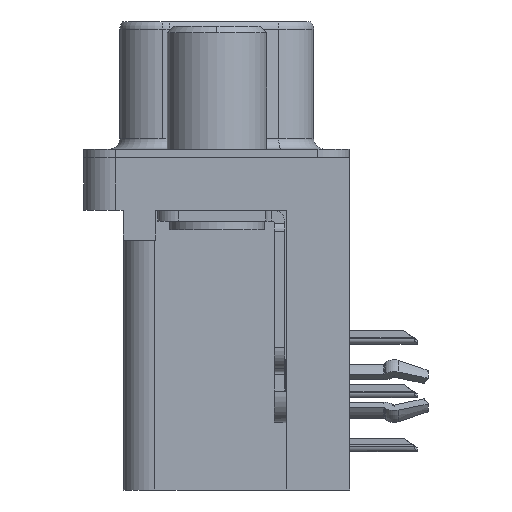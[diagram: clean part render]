
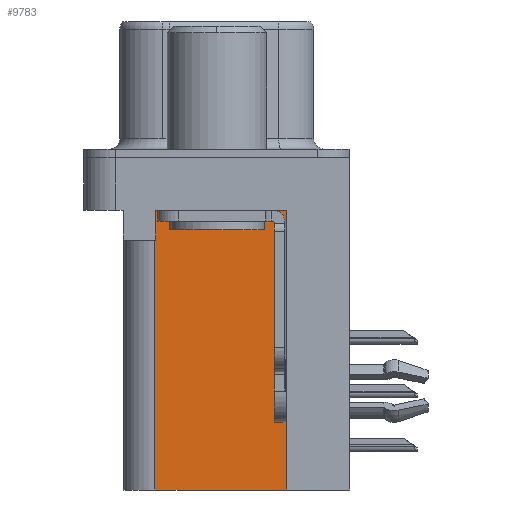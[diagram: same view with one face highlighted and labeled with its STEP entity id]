
A CAD part, left-side view. The second image highlights one B-rep face of the part: STEP entity #9783.
In plain terms, the highlighted planar face has unit normal (-1, 0, 0).
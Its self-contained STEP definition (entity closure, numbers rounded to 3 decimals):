
#446 = LINE ( 'NONE', #5777, #25741 ) ;
#707 = DIRECTION ( 'NONE',  ( 0., 1., 0. ) ) ;
#955 = EDGE_CURVE ( 'NONE', #17339, #7698, #11703, .T. ) ;
#1466 = CARTESIAN_POINT ( 'NONE',  ( 3.7, 2.895, -3.9 ) ) ;
#1487 = VECTOR ( 'NONE', #15328, 1000. ) ;
#1498 = CARTESIAN_POINT ( 'NONE',  ( 3.7, -3.295, -2.5 ) ) ;
#1516 = CARTESIAN_POINT ( 'NONE',  ( 3.7, -3.295, -15.7 ) ) ;
#1815 = EDGE_LOOP ( 'NONE', ( #8697, #21644, #10658, #1961, #14546, #3160 ) ) ;
#1961 = ORIENTED_EDGE ( 'NONE', *, *, #21265, .F. ) ;
#2365 = LINE ( 'NONE', #6939, #14614 ) ;
#3116 = CARTESIAN_POINT ( 'NONE',  ( 3.7, -3.295, -15.7 ) ) ;
#3160 = ORIENTED_EDGE ( 'NONE', *, *, #5822, .T. ) ;
#4109 = EDGE_CURVE ( 'NONE', #21103, #10882, #446, .T. ) ;
#4469 = LINE ( 'NONE', #10552, #9457 ) ;
#5218 = VECTOR ( 'NONE', #707, 1000. ) ;
#5386 = CARTESIAN_POINT ( 'NONE',  ( 3.7, 0., -3.9 ) ) ;
#5605 = VERTEX_POINT ( 'NONE', #7280 ) ;
#5777 = CARTESIAN_POINT ( 'NONE',  ( 3.7, -3.295, -15.7 ) ) ;
#5822 = EDGE_CURVE ( 'NONE', #21103, #17487, #21041, .T. ) ;
#6395 = DIRECTION ( 'NONE',  ( 0., 1., 0. ) ) ;
#6939 = CARTESIAN_POINT ( 'NONE',  ( 3.7, 2.925, -15.7 ) ) ;
#7280 = CARTESIAN_POINT ( 'NONE',  ( 3.7, 2.895, -2.5 ) ) ;
#7698 = VERTEX_POINT ( 'NONE', #30612 ) ;
#8006 = AXIS2_PLACEMENT_3D ( 'NONE', #19980, #10215, #27384 ) ;
#8697 = ORIENTED_EDGE ( 'NONE', *, *, #16699, .T. ) ;
#9457 = VECTOR ( 'NONE', #13104, 1000. ) ;
#9783 = ADVANCED_FACE ( 'NONE', ( #30128 ), #29740, .F. ) ;
#10215 = DIRECTION ( 'NONE',  ( 1., 0., 0. ) ) ;
#10552 = CARTESIAN_POINT ( 'NONE',  ( 3.7, 2.895, -3.9 ) ) ;
#10658 = ORIENTED_EDGE ( 'NONE', *, *, #955, .T. ) ;
#10702 = DIRECTION ( 'NONE',  ( 0., 1., 0. ) ) ;
#10882 = VERTEX_POINT ( 'NONE', #17533 ) ;
#11703 = LINE ( 'NONE', #5386, #5218 ) ;
#13104 = DIRECTION ( 'NONE',  ( 0., 0., -1. ) ) ;
#14546 = ORIENTED_EDGE ( 'NONE', *, *, #4109, .F. ) ;
#14614 = VECTOR ( 'NONE', #31694, 1000. ) ;
#15328 = DIRECTION ( 'NONE',  ( 0., 0., 1. ) ) ;
#15543 = VECTOR ( 'NONE', #6395, 1000. ) ;
#16305 = LINE ( 'NONE', #1498, #15543 ) ;
#16699 = EDGE_CURVE ( 'NONE', #17487, #5605, #16305, .T. ) ;
#17339 = VERTEX_POINT ( 'NONE', #1466 ) ;
#17487 = VERTEX_POINT ( 'NONE', #19222 ) ;
#17533 = CARTESIAN_POINT ( 'NONE',  ( 3.7, 2.925, -15.7 ) ) ;
#19222 = CARTESIAN_POINT ( 'NONE',  ( 3.7, -3.295, -2.5 ) ) ;
#19980 = CARTESIAN_POINT ( 'NONE',  ( 3.7, -3.295, -15.7 ) ) ;
#21041 = LINE ( 'NONE', #3116, #1487 ) ;
#21103 = VERTEX_POINT ( 'NONE', #1516 ) ;
#21265 = EDGE_CURVE ( 'NONE', #10882, #7698, #2365, .T. ) ;
#21644 = ORIENTED_EDGE ( 'NONE', *, *, #24041, .T. ) ;
#24041 = EDGE_CURVE ( 'NONE', #5605, #17339, #4469, .T. ) ;
#25741 = VECTOR ( 'NONE', #10702, 1000. ) ;
#27384 = DIRECTION ( 'NONE',  ( 0., 0., -1. ) ) ;
#29740 = PLANE ( 'NONE',  #8006 ) ;
#30128 = FACE_OUTER_BOUND ( 'NONE', #1815, .T. ) ;
#30612 = CARTESIAN_POINT ( 'NONE',  ( 3.7, 2.925, -3.9 ) ) ;
#31694 = DIRECTION ( 'NONE',  ( 0., 0., 1. ) ) ;
